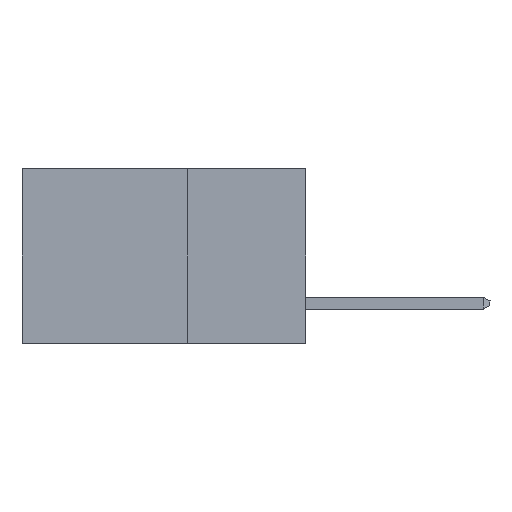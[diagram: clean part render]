
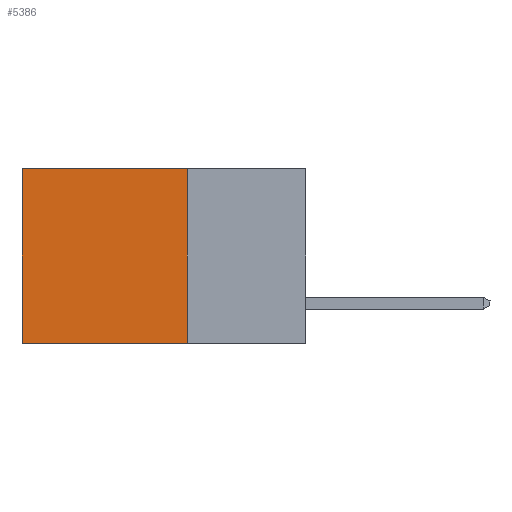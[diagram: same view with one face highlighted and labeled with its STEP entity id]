
A CAD part, left-side view. The second image highlights one B-rep face of the part: STEP entity #5386.
In plain terms, the highlighted planar face has unit normal (-1, 0, 0).
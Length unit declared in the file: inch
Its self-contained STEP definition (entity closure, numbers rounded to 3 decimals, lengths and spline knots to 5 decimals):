
#133 = VECTOR ( 'NONE', #10166, 39.37008 ) ;
#813 = EDGE_LOOP ( 'NONE', ( #10823, #969, #5424, #32051 ) ) ;
#969 = ORIENTED_EDGE ( 'NONE', *, *, #12099, .F. ) ;
#4437 = LINE ( 'NONE', #12084, #27132 ) ;
#4449 = VECTOR ( 'NONE', #31916, 39.37008 ) ;
#4561 = VERTEX_POINT ( 'NONE', #28695 ) ;
#4582 = PLANE ( 'NONE',  #26068 ) ;
#5386 = ADVANCED_FACE ( 'NONE', ( #5828 ), #4582, .F. ) ;
#5388 = VERTEX_POINT ( 'NONE', #21869 ) ;
#5424 = ORIENTED_EDGE ( 'NONE', *, *, #29634, .F. ) ;
#5828 = FACE_OUTER_BOUND ( 'NONE', #813, .T. ) ;
#9098 = CARTESIAN_POINT ( 'NONE',  ( 0.298, 0.6, 0. ) ) ;
#10166 = DIRECTION ( 'NONE',  ( 0., 1., 0. ) ) ;
#10823 = ORIENTED_EDGE ( 'NONE', *, *, #30360, .T. ) ;
#12084 = CARTESIAN_POINT ( 'NONE',  ( 0.298, 0.25, -0.37 ) ) ;
#12099 = EDGE_CURVE ( 'NONE', #31912, #4561, #4437, .T. ) ;
#12669 = LINE ( 'NONE', #9098, #4449 ) ;
#15755 = CARTESIAN_POINT ( 'NONE',  ( 0.298, 0.25, 0. ) ) ;
#16606 = LINE ( 'NONE', #15755, #29109 ) ;
#17167 = CARTESIAN_POINT ( 'NONE',  ( 0.298, 0.25, 0. ) ) ;
#17564 = CARTESIAN_POINT ( 'NONE',  ( 0.298, 0.25, -0.37 ) ) ;
#20809 = DIRECTION ( 'NONE',  ( 0., 0., -1. ) ) ;
#21869 = CARTESIAN_POINT ( 'NONE',  ( 0.298, 0.6, 0. ) ) ;
#22098 = DIRECTION ( 'NONE',  ( 0., 0., -1. ) ) ;
#22561 = CARTESIAN_POINT ( 'NONE',  ( 0.298, 0.25, 0. ) ) ;
#23667 = LINE ( 'NONE', #22561, #133 ) ;
#24320 = VERTEX_POINT ( 'NONE', #25198 ) ;
#25198 = CARTESIAN_POINT ( 'NONE',  ( 0.298, 0.25, 0. ) ) ;
#26068 = AXIS2_PLACEMENT_3D ( 'NONE', #17167, #29300, #22098 ) ;
#26755 = EDGE_CURVE ( 'NONE', #24320, #5388, #23667, .T. ) ;
#27132 = VECTOR ( 'NONE', #29611, 39.37008 ) ;
#28695 = CARTESIAN_POINT ( 'NONE',  ( 0.298, 0.6, -0.37 ) ) ;
#29109 = VECTOR ( 'NONE', #20809, 39.37008 ) ;
#29300 = DIRECTION ( 'NONE',  ( 1., 0., 0. ) ) ;
#29611 = DIRECTION ( 'NONE',  ( 0., 1., 0. ) ) ;
#29634 = EDGE_CURVE ( 'NONE', #24320, #31912, #16606, .T. ) ;
#30360 = EDGE_CURVE ( 'NONE', #5388, #4561, #12669, .T. ) ;
#31912 = VERTEX_POINT ( 'NONE', #17564 ) ;
#31916 = DIRECTION ( 'NONE',  ( 0., 0., -1. ) ) ;
#32051 = ORIENTED_EDGE ( 'NONE', *, *, #26755, .T. ) ;
